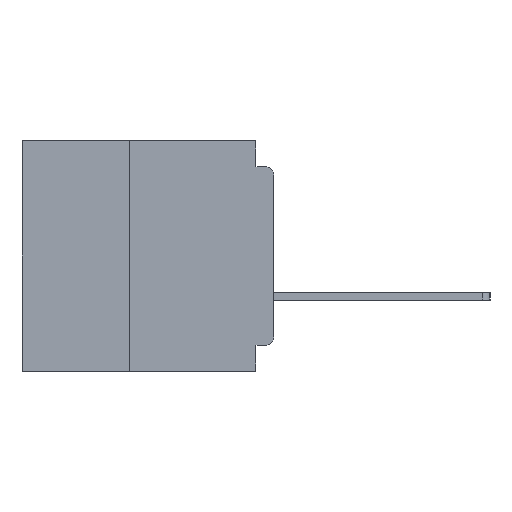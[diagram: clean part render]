
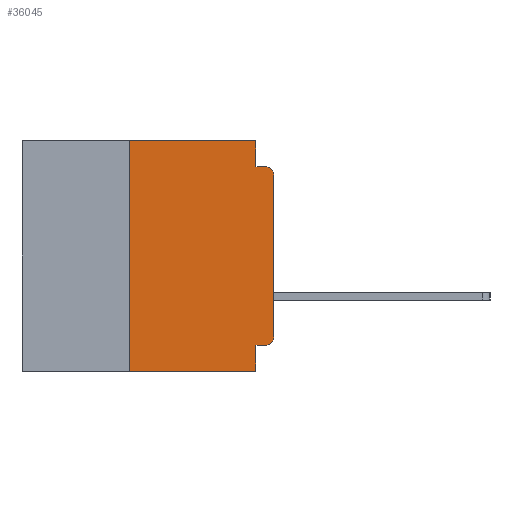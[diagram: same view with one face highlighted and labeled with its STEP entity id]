
A CAD part, left-side view. The second image highlights one B-rep face of the part: STEP entity #36045.
In plain terms, the highlighted planar face has unit normal (-1, 0, 0).
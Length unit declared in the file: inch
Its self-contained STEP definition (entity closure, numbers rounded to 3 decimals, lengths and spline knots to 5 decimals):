
#147 = CARTESIAN_POINT ( 'NONE',  ( 0., 0., -0.06 ) ) ;
#1204 = VERTEX_POINT ( 'NONE', #147 ) ;
#1332 = CARTESIAN_POINT ( 'NONE',  ( 0., 0.031, -0.355 ) ) ;
#1952 = DIRECTION ( 'NONE',  ( 0., 0., -1. ) ) ;
#2291 = DIRECTION ( 'NONE',  ( 1., 0., 0. ) ) ;
#2965 = VERTEX_POINT ( 'NONE', #36487 ) ;
#3817 = EDGE_CURVE ( 'NONE', #29294, #11825, #14617, .T. ) ;
#4062 = LINE ( 'NONE', #33628, #34408 ) ;
#4200 = CARTESIAN_POINT ( 'NONE',  ( 0., 0.015, -0.045 ) ) ;
#4300 = VECTOR ( 'NONE', #28342, 39.37008 ) ;
#4378 = VERTEX_POINT ( 'NONE', #22472 ) ;
#4957 = CARTESIAN_POINT ( 'NONE',  ( 0., 0.25, -0.4 ) ) ;
#5230 = LINE ( 'NONE', #22207, #4300 ) ;
#5519 = ORIENTED_EDGE ( 'NONE', *, *, #16176, .F. ) ;
#6037 = ORIENTED_EDGE ( 'NONE', *, *, #37547, .T. ) ;
#6557 = VECTOR ( 'NONE', #31820, 39.37008 ) ;
#7236 = FACE_OUTER_BOUND ( 'NONE', #8134, .T. ) ;
#7279 = AXIS2_PLACEMENT_3D ( 'NONE', #38199, #20075, #1952 ) ;
#8128 = EDGE_CURVE ( 'NONE', #11825, #4378, #11008, .T. ) ;
#8134 = EDGE_LOOP ( 'NONE', ( #25499, #24723, #21933, #21538, #5519, #33376, #35594, #23311, #16252, #6037 ) ) ;
#8142 = VERTEX_POINT ( 'NONE', #20395 ) ;
#9682 = VERTEX_POINT ( 'NONE', #21755 ) ;
#11008 = LINE ( 'NONE', #32508, #35233 ) ;
#11725 = DIRECTION ( 'NONE',  ( -1., 0., 0. ) ) ;
#11825 = VERTEX_POINT ( 'NONE', #1332 ) ;
#12523 = LINE ( 'NONE', #30026, #36727 ) ;
#13486 = CARTESIAN_POINT ( 'NONE',  ( 0., 0.25, -0.4 ) ) ;
#14040 = EDGE_CURVE ( 'NONE', #9682, #1204, #12523, .T. ) ;
#14305 = DIRECTION ( 'NONE',  ( 0., 0., -1. ) ) ;
#14454 = VECTOR ( 'NONE', #31107, 39.37008 ) ;
#14617 = LINE ( 'NONE', #34853, #6557 ) ;
#16176 = EDGE_CURVE ( 'NONE', #2965, #8142, #5230, .T. ) ;
#16252 = ORIENTED_EDGE ( 'NONE', *, *, #3817, .F. ) ;
#16476 = CIRCLE ( 'NONE', #20279, 0.015 ) ;
#17303 = LINE ( 'NONE', #35924, #18239 ) ;
#17369 = VERTEX_POINT ( 'NONE', #13486 ) ;
#17398 = PLANE ( 'NONE',  #26142 ) ;
#17902 = VERTEX_POINT ( 'NONE', #4200 ) ;
#18239 = VECTOR ( 'NONE', #38867, 39.37008 ) ;
#18857 = CARTESIAN_POINT ( 'NONE',  ( 0., 0.437, -0.4 ) ) ;
#19286 = EDGE_CURVE ( 'NONE', #22016, #17902, #17303, .T. ) ;
#20075 = DIRECTION ( 'NONE',  ( -1., 0., 0. ) ) ;
#20173 = DIRECTION ( 'NONE',  ( 0., 0., 1. ) ) ;
#20279 = AXIS2_PLACEMENT_3D ( 'NONE', #29965, #11725, #32984 ) ;
#20395 = CARTESIAN_POINT ( 'NONE',  ( 0., 0.031, 0. ) ) ;
#20431 = CARTESIAN_POINT ( 'NONE',  ( 0., 0.437, 0. ) ) ;
#21029 = CIRCLE ( 'NONE', #7279, 0.015 ) ;
#21522 = DIRECTION ( 'NONE',  ( 0., 0., -1. ) ) ;
#21538 = ORIENTED_EDGE ( 'NONE', *, *, #34032, .F. ) ;
#21755 = CARTESIAN_POINT ( 'NONE',  ( 0., 0., -0.34 ) ) ;
#21933 = ORIENTED_EDGE ( 'NONE', *, *, #19286, .F. ) ;
#22016 = VERTEX_POINT ( 'NONE', #31099 ) ;
#22207 = CARTESIAN_POINT ( 'NONE',  ( 0., 0.437, 0. ) ) ;
#22472 = CARTESIAN_POINT ( 'NONE',  ( 0., 0.031, -0.4 ) ) ;
#22522 = LINE ( 'NONE', #18857, #14454 ) ;
#23311 = ORIENTED_EDGE ( 'NONE', *, *, #8128, .F. ) ;
#23499 = DIRECTION ( 'NONE',  ( 0., 0., -1. ) ) ;
#23512 = CARTESIAN_POINT ( 'NONE',  ( 0., 0.015, -0.355 ) ) ;
#24723 = ORIENTED_EDGE ( 'NONE', *, *, #35460, .T. ) ;
#25499 = ORIENTED_EDGE ( 'NONE', *, *, #14040, .T. ) ;
#26142 = AXIS2_PLACEMENT_3D ( 'NONE', #20431, #2291, #23499 ) ;
#28342 = DIRECTION ( 'NONE',  ( 0., -1., 0. ) ) ;
#28798 = VECTOR ( 'NONE', #20173, 39.37008 ) ;
#29294 = VERTEX_POINT ( 'NONE', #23512 ) ;
#29754 = LINE ( 'NONE', #4957, #28798 ) ;
#29965 = CARTESIAN_POINT ( 'NONE',  ( 0., 0.015, -0.34 ) ) ;
#30026 = CARTESIAN_POINT ( 'NONE',  ( 0., 0., 0. ) ) ;
#31099 = CARTESIAN_POINT ( 'NONE',  ( 0., 0.031, -0.045 ) ) ;
#31107 = DIRECTION ( 'NONE',  ( 0., -1., 0. ) ) ;
#31820 = DIRECTION ( 'NONE',  ( 0., 1., 0. ) ) ;
#32508 = CARTESIAN_POINT ( 'NONE',  ( 0., 0.031, -0.4 ) ) ;
#32984 = DIRECTION ( 'NONE',  ( 0., 0., -1. ) ) ;
#33376 = ORIENTED_EDGE ( 'NONE', *, *, #38050, .F. ) ;
#33628 = CARTESIAN_POINT ( 'NONE',  ( 0., 0.031, 0. ) ) ;
#34032 = EDGE_CURVE ( 'NONE', #8142, #22016, #4062, .T. ) ;
#34131 = EDGE_CURVE ( 'NONE', #17369, #4378, #22522, .T. ) ;
#34408 = VECTOR ( 'NONE', #21522, 39.37008 ) ;
#34853 = CARTESIAN_POINT ( 'NONE',  ( 0., 0., -0.355 ) ) ;
#35233 = VECTOR ( 'NONE', #14305, 39.37008 ) ;
#35460 = EDGE_CURVE ( 'NONE', #1204, #17902, #21029, .T. ) ;
#35594 = ORIENTED_EDGE ( 'NONE', *, *, #34131, .T. ) ;
#35924 = CARTESIAN_POINT ( 'NONE',  ( 0., 0., -0.045 ) ) ;
#36045 = ADVANCED_FACE ( 'NONE', ( #7236 ), #17398, .F. ) ;
#36487 = CARTESIAN_POINT ( 'NONE',  ( 0., 0.25, 0. ) ) ;
#36727 = VECTOR ( 'NONE', #39016, 39.37008 ) ;
#37547 = EDGE_CURVE ( 'NONE', #29294, #9682, #16476, .T. ) ;
#38050 = EDGE_CURVE ( 'NONE', #17369, #2965, #29754, .T. ) ;
#38199 = CARTESIAN_POINT ( 'NONE',  ( 0., 0.015, -0.06 ) ) ;
#38867 = DIRECTION ( 'NONE',  ( 0., -1., 0. ) ) ;
#39016 = DIRECTION ( 'NONE',  ( 0., 0., 1. ) ) ;
